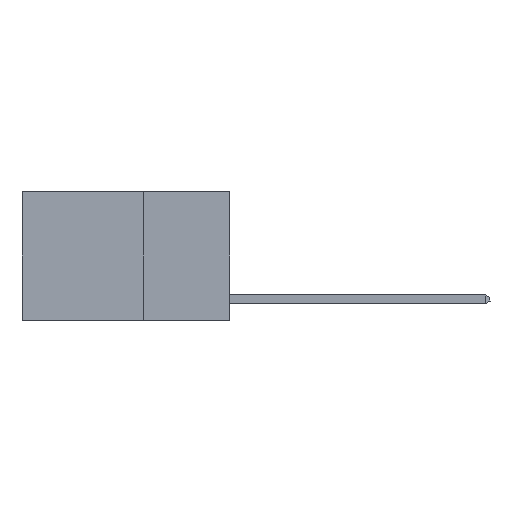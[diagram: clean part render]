
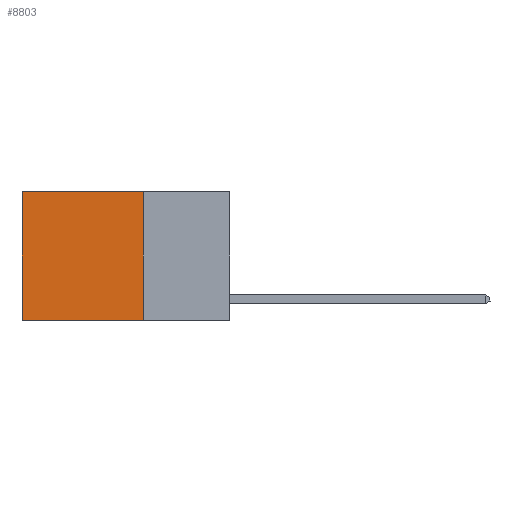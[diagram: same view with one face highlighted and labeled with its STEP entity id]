
A CAD part, left-side view. The second image highlights one B-rep face of the part: STEP entity #8803.
In plain terms, the highlighted planar face has unit normal (-1, 0, 0).
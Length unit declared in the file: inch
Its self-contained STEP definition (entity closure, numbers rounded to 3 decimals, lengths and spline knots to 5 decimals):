
#38 = EDGE_LOOP ( 'NONE', ( #3954, #3411, #3194, #3497 ) ) ;
#275 = CARTESIAN_POINT ( 'NONE',  ( 0.2625, 0.25, 0. ) ) ;
#680 = LINE ( 'NONE', #7330, #10290 ) ;
#1026 = EDGE_CURVE ( 'NONE', #11276, #4720, #680, .T. ) ;
#1465 = CARTESIAN_POINT ( 'NONE',  ( 0.2625, 0.6, 0. ) ) ;
#1644 = FACE_OUTER_BOUND ( 'NONE', #38, .T. ) ;
#2381 = CARTESIAN_POINT ( 'NONE',  ( 0.2625, 0.6, 0. ) ) ;
#2813 = VERTEX_POINT ( 'NONE', #1465 ) ;
#3194 = ORIENTED_EDGE ( 'NONE', *, *, #6677, .F. ) ;
#3217 = CARTESIAN_POINT ( 'NONE',  ( 0.2625, 0.25, 0. ) ) ;
#3411 = ORIENTED_EDGE ( 'NONE', *, *, #1026, .F. ) ;
#3437 = LINE ( 'NONE', #2381, #6343 ) ;
#3497 = ORIENTED_EDGE ( 'NONE', *, *, #7100, .T. ) ;
#3954 = ORIENTED_EDGE ( 'NONE', *, *, #9551, .T. ) ;
#4443 = DIRECTION ( 'NONE',  ( 0., 0., -1. ) ) ;
#4720 = VERTEX_POINT ( 'NONE', #11064 ) ;
#5314 = CARTESIAN_POINT ( 'NONE',  ( 0.2625, 0.25, -0.37 ) ) ;
#5486 = DIRECTION ( 'NONE',  ( 0., 0., -1. ) ) ;
#5975 = LINE ( 'NONE', #9002, #9515 ) ;
#6284 = DIRECTION ( 'NONE',  ( 0., 1., 0. ) ) ;
#6343 = VECTOR ( 'NONE', #4443, 39.37008 ) ;
#6677 = EDGE_CURVE ( 'NONE', #10259, #11276, #8200, .T. ) ;
#7100 = EDGE_CURVE ( 'NONE', #10259, #2813, #5975, .T. ) ;
#7330 = CARTESIAN_POINT ( 'NONE',  ( 0.2625, 0.25, -0.37 ) ) ;
#7748 = AXIS2_PLACEMENT_3D ( 'NONE', #12354, #9421, #5486 ) ;
#8004 = DIRECTION ( 'NONE',  ( 0., 1., 0. ) ) ;
#8018 = DIRECTION ( 'NONE',  ( 0., 0., -1. ) ) ;
#8200 = LINE ( 'NONE', #275, #12097 ) ;
#8803 = ADVANCED_FACE ( 'NONE', ( #1644 ), #10281, .F. ) ;
#9002 = CARTESIAN_POINT ( 'NONE',  ( 0.2625, 0.25, 0. ) ) ;
#9421 = DIRECTION ( 'NONE',  ( 1., 0., 0. ) ) ;
#9515 = VECTOR ( 'NONE', #8004, 39.37008 ) ;
#9551 = EDGE_CURVE ( 'NONE', #2813, #4720, #3437, .T. ) ;
#10259 = VERTEX_POINT ( 'NONE', #3217 ) ;
#10281 = PLANE ( 'NONE',  #7748 ) ;
#10290 = VECTOR ( 'NONE', #6284, 39.37008 ) ;
#11064 = CARTESIAN_POINT ( 'NONE',  ( 0.2625, 0.6, -0.37 ) ) ;
#11276 = VERTEX_POINT ( 'NONE', #5314 ) ;
#12097 = VECTOR ( 'NONE', #8018, 39.37008 ) ;
#12354 = CARTESIAN_POINT ( 'NONE',  ( 0.2625, 0.25, 0. ) ) ;
